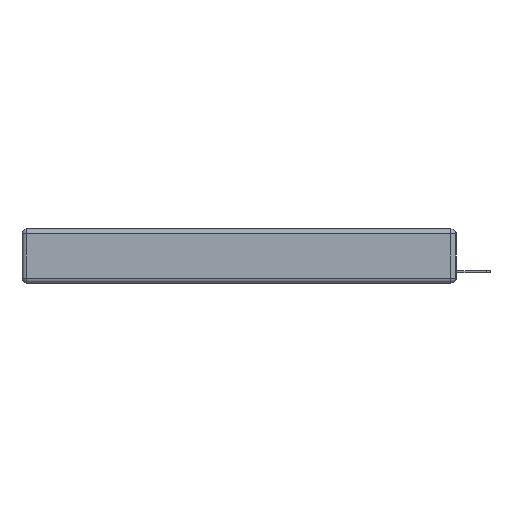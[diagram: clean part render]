
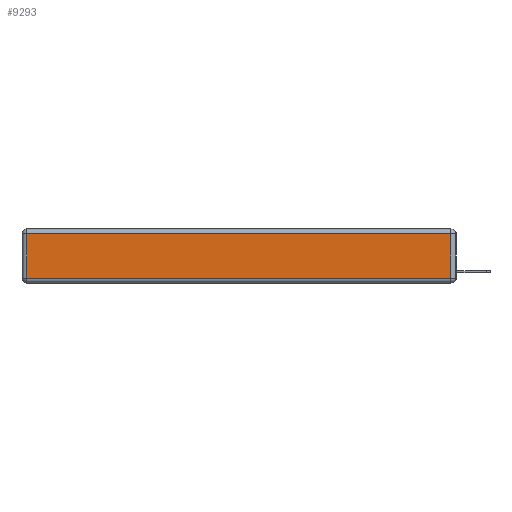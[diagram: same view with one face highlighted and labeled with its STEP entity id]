
A CAD part, left-side view. The second image highlights one B-rep face of the part: STEP entity #9293.
In plain terms, the highlighted planar face has unit normal (-1, 0, 0).
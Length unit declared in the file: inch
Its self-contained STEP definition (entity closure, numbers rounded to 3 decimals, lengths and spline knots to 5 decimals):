
#1089 = DIRECTION ( 'NONE',  ( 0., 0., -1. ) ) ;
#1178 = ORIENTED_EDGE ( 'NONE', *, *, #7955, .T. ) ;
#1242 = ORIENTED_EDGE ( 'NONE', *, *, #5466, .T. ) ;
#1395 = CARTESIAN_POINT ( 'NONE',  ( 0., 2.72, -0.313 ) ) ;
#1928 = FACE_OUTER_BOUND ( 'NONE', #7291, .T. ) ;
#2809 = DIRECTION ( 'NONE',  ( 0., 0., 1. ) ) ;
#2911 = VERTEX_POINT ( 'NONE', #8920 ) ;
#3295 = LINE ( 'NONE', #8260, #9821 ) ;
#3404 = CARTESIAN_POINT ( 'NONE',  ( 0., 0.03, -0.343 ) ) ;
#3779 = CARTESIAN_POINT ( 'NONE',  ( 0., 0., -0.343 ) ) ;
#3875 = VECTOR ( 'NONE', #1089, 39.37008 ) ;
#4562 = EDGE_CURVE ( 'NONE', #2911, #5147, #3295, .T. ) ;
#4633 = CARTESIAN_POINT ( 'NONE',  ( 0., 0.03, -0.313 ) ) ;
#4691 = ORIENTED_EDGE ( 'NONE', *, *, #4562, .T. ) ;
#4790 = CARTESIAN_POINT ( 'NONE',  ( 0., 2.72, -0.03 ) ) ;
#4959 = LINE ( 'NONE', #3404, #12949 ) ;
#5147 = VERTEX_POINT ( 'NONE', #4790 ) ;
#5466 = EDGE_CURVE ( 'NONE', #12102, #2911, #4959, .T. ) ;
#5950 = DIRECTION ( 'NONE',  ( -1., 0., 0. ) ) ;
#6456 = CARTESIAN_POINT ( 'NONE',  ( 0., 2.72, -0.343 ) ) ;
#6920 = CARTESIAN_POINT ( 'NONE',  ( 0., 0., -0.313 ) ) ;
#7014 = LINE ( 'NONE', #6920, #9325 ) ;
#7068 = DIRECTION ( 'NONE',  ( 0., 1., 0. ) ) ;
#7291 = EDGE_LOOP ( 'NONE', ( #1178, #1242, #4691, #10433 ) ) ;
#7955 = EDGE_CURVE ( 'NONE', #12503, #12102, #7014, .T. ) ;
#8036 = DIRECTION ( 'NONE',  ( 0., -1., 0. ) ) ;
#8260 = CARTESIAN_POINT ( 'NONE',  ( 0., 2.75, -0.03 ) ) ;
#8572 = AXIS2_PLACEMENT_3D ( 'NONE', #3779, #5950, #2809 ) ;
#8920 = CARTESIAN_POINT ( 'NONE',  ( 0., 0.03, -0.03 ) ) ;
#9293 = ADVANCED_FACE ( 'NONE', ( #1928 ), #10169, .T. ) ;
#9325 = VECTOR ( 'NONE', #8036, 39.37008 ) ;
#9821 = VECTOR ( 'NONE', #7068, 39.37008 ) ;
#10169 = PLANE ( 'NONE',  #8572 ) ;
#10433 = ORIENTED_EDGE ( 'NONE', *, *, #10630, .T. ) ;
#10630 = EDGE_CURVE ( 'NONE', #5147, #12503, #10719, .T. ) ;
#10719 = LINE ( 'NONE', #6456, #3875 ) ;
#11935 = DIRECTION ( 'NONE',  ( 0., 0., 1. ) ) ;
#12102 = VERTEX_POINT ( 'NONE', #4633 ) ;
#12503 = VERTEX_POINT ( 'NONE', #1395 ) ;
#12949 = VECTOR ( 'NONE', #11935, 39.37008 ) ;
